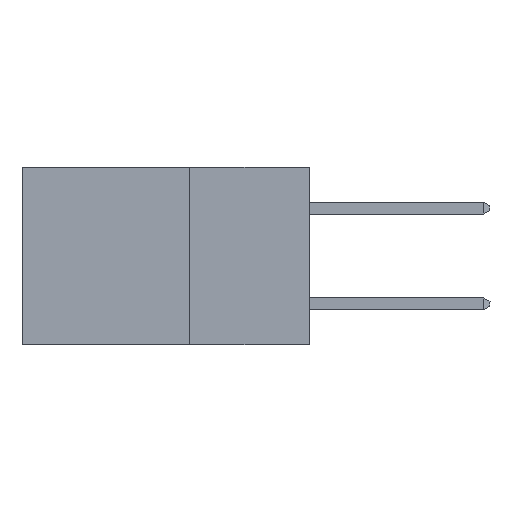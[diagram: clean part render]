
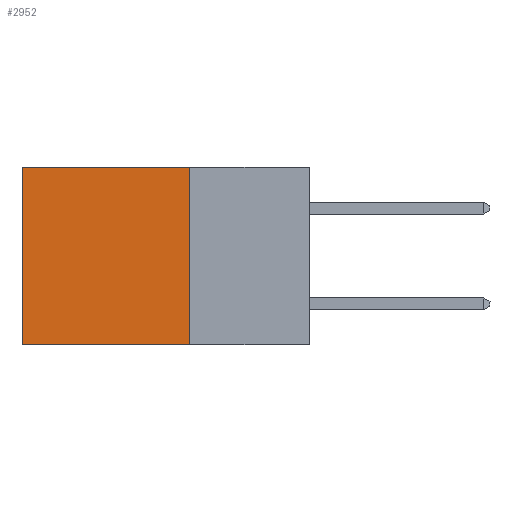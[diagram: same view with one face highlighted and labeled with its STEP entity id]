
A CAD part, left-side view. The second image highlights one B-rep face of the part: STEP entity #2952.
In plain terms, the highlighted planar face has unit normal (-1, 0, 0).
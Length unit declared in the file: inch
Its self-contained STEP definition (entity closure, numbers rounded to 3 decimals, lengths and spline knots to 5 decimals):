
#17 = CARTESIAN_POINT ( 'NONE',  ( 0.2875, 0.25, 0. ) ) ;
#135 = LINE ( 'NONE', #250, #10953 ) ;
#250 = CARTESIAN_POINT ( 'NONE',  ( 0.2875, 0.25, 0. ) ) ;
#437 = CARTESIAN_POINT ( 'NONE',  ( 0.2875, 0.25, 0. ) ) ;
#555 = LINE ( 'NONE', #437, #8506 ) ;
#694 = DIRECTION ( 'NONE',  ( 0., 1., 0. ) ) ;
#1164 = VERTEX_POINT ( 'NONE', #8978 ) ;
#1280 = AXIS2_PLACEMENT_3D ( 'NONE', #2550, #6224, #9930 ) ;
#1471 = CARTESIAN_POINT ( 'NONE',  ( 0.2875, 0.25, -0.37 ) ) ;
#1872 = EDGE_CURVE ( 'NONE', #1164, #5786, #6933, .T. ) ;
#2316 = PLANE ( 'NONE',  #1280 ) ;
#2341 = DIRECTION ( 'NONE',  ( 0., 0., -1. ) ) ;
#2430 = VECTOR ( 'NONE', #694, 39.37008 ) ;
#2550 = CARTESIAN_POINT ( 'NONE',  ( 0.2875, 0.25, 0. ) ) ;
#2872 = EDGE_CURVE ( 'NONE', #11112, #5786, #7931, .T. ) ;
#2952 = ADVANCED_FACE ( 'NONE', ( #9811 ), #2316, .F. ) ;
#4092 = ORIENTED_EDGE ( 'NONE', *, *, #1872, .T. ) ;
#5786 = VERTEX_POINT ( 'NONE', #11583 ) ;
#6224 = DIRECTION ( 'NONE',  ( 1., 0., 0. ) ) ;
#6933 = LINE ( 'NONE', #10636, #7986 ) ;
#7755 = ORIENTED_EDGE ( 'NONE', *, *, #2872, .F. ) ;
#7931 = LINE ( 'NONE', #1471, #2430 ) ;
#7986 = VECTOR ( 'NONE', #2341, 39.37008 ) ;
#8416 = EDGE_CURVE ( 'NONE', #9584, #11112, #135, .T. ) ;
#8506 = VECTOR ( 'NONE', #9784, 39.37008 ) ;
#8978 = CARTESIAN_POINT ( 'NONE',  ( 0.2875, 0.6, 0. ) ) ;
#9584 = VERTEX_POINT ( 'NONE', #17 ) ;
#9784 = DIRECTION ( 'NONE',  ( 0., 1., 0. ) ) ;
#9811 = FACE_OUTER_BOUND ( 'NONE', #11673, .T. ) ;
#9930 = DIRECTION ( 'NONE',  ( 0., 0., -1. ) ) ;
#10375 = ORIENTED_EDGE ( 'NONE', *, *, #8416, .F. ) ;
#10636 = CARTESIAN_POINT ( 'NONE',  ( 0.2875, 0.6, 0. ) ) ;
#10760 = CARTESIAN_POINT ( 'NONE',  ( 0.2875, 0.25, -0.37 ) ) ;
#10810 = ORIENTED_EDGE ( 'NONE', *, *, #11166, .T. ) ;
#10953 = VECTOR ( 'NONE', #11321, 39.37008 ) ;
#11112 = VERTEX_POINT ( 'NONE', #10760 ) ;
#11166 = EDGE_CURVE ( 'NONE', #9584, #1164, #555, .T. ) ;
#11321 = DIRECTION ( 'NONE',  ( 0., 0., -1. ) ) ;
#11583 = CARTESIAN_POINT ( 'NONE',  ( 0.2875, 0.6, -0.37 ) ) ;
#11673 = EDGE_LOOP ( 'NONE', ( #4092, #7755, #10375, #10810 ) ) ;
